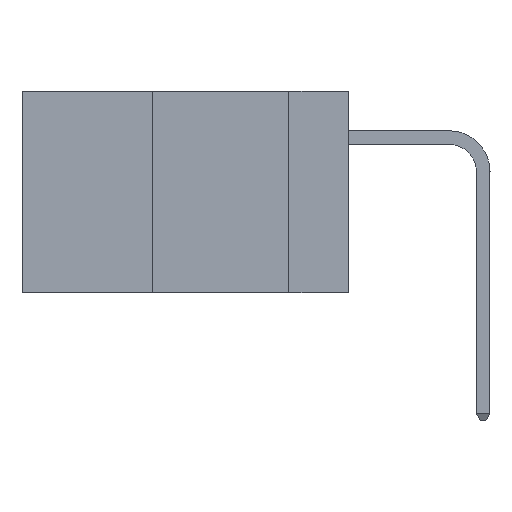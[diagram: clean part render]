
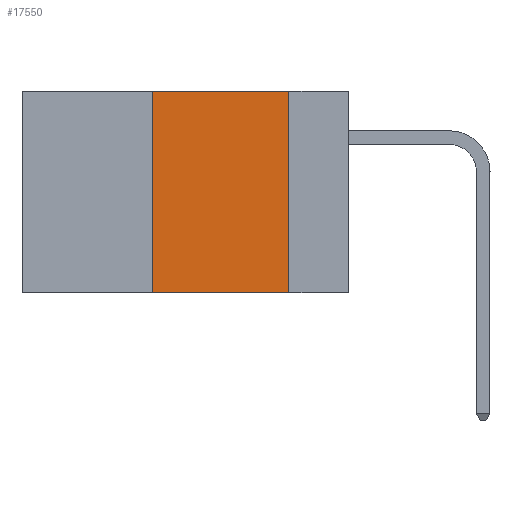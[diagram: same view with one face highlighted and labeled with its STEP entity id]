
A CAD part, left-side view. The second image highlights one B-rep face of the part: STEP entity #17550.
In plain terms, the highlighted planar face has unit normal (-1, 0, 0).
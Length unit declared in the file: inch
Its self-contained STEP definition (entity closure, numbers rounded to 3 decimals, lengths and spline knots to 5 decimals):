
#295 = CARTESIAN_POINT ( 'NONE',  ( 0., 0.6, 0. ) ) ;
#1235 = CARTESIAN_POINT ( 'NONE',  ( 0., 0.11, 0. ) ) ;
#1317 = LINE ( 'NONE', #26488, #11459 ) ;
#2123 = VECTOR ( 'NONE', #9400, 39.37008 ) ;
#2427 = AXIS2_PLACEMENT_3D ( 'NONE', #295, #12502, #10714 ) ;
#2477 = CARTESIAN_POINT ( 'NONE',  ( 0., 0.11, -0.37 ) ) ;
#3123 = CARTESIAN_POINT ( 'NONE',  ( 0., 0.36, 0. ) ) ;
#3642 = CARTESIAN_POINT ( 'NONE',  ( 0., 0.36, -0.37 ) ) ;
#4327 = DIRECTION ( 'NONE',  ( 0., 0., -1. ) ) ;
#4643 = ORIENTED_EDGE ( 'NONE', *, *, #7708, .F. ) ;
#5728 = VERTEX_POINT ( 'NONE', #2477 ) ;
#7194 = ORIENTED_EDGE ( 'NONE', *, *, #15128, .T. ) ;
#7613 = VECTOR ( 'NONE', #17312, 39.37008 ) ;
#7708 = EDGE_CURVE ( 'NONE', #18849, #19179, #10596, .T. ) ;
#8926 = LINE ( 'NONE', #25757, #7613 ) ;
#9400 = DIRECTION ( 'NONE',  ( 0., 0., 1. ) ) ;
#9560 = EDGE_CURVE ( 'NONE', #19179, #5728, #1317, .T. ) ;
#10142 = DIRECTION ( 'NONE',  ( 0., -1., 0. ) ) ;
#10240 = CARTESIAN_POINT ( 'NONE',  ( 0., 0.6, 0. ) ) ;
#10596 = LINE ( 'NONE', #10240, #25767 ) ;
#10714 = DIRECTION ( 'NONE',  ( 0., 0., -1. ) ) ;
#11459 = VECTOR ( 'NONE', #4327, 39.37008 ) ;
#11768 = ORIENTED_EDGE ( 'NONE', *, *, #9560, .F. ) ;
#11888 = VERTEX_POINT ( 'NONE', #3642 ) ;
#12502 = DIRECTION ( 'NONE',  ( 1., 0., 0. ) ) ;
#15128 = EDGE_CURVE ( 'NONE', #11888, #5728, #8926, .T. ) ;
#16936 = FACE_OUTER_BOUND ( 'NONE', #25085, .T. ) ;
#17312 = DIRECTION ( 'NONE',  ( 0., -1., 0. ) ) ;
#17407 = LINE ( 'NONE', #3123, #2123 ) ;
#17550 = ADVANCED_FACE ( 'NONE', ( #16936 ), #24887, .F. ) ;
#18849 = VERTEX_POINT ( 'NONE', #22954 ) ;
#19179 = VERTEX_POINT ( 'NONE', #1235 ) ;
#22390 = EDGE_CURVE ( 'NONE', #11888, #18849, #17407, .T. ) ;
#22954 = CARTESIAN_POINT ( 'NONE',  ( 0., 0.36, 0. ) ) ;
#23325 = ORIENTED_EDGE ( 'NONE', *, *, #22390, .F. ) ;
#24887 = PLANE ( 'NONE',  #2427 ) ;
#25085 = EDGE_LOOP ( 'NONE', ( #11768, #4643, #23325, #7194 ) ) ;
#25757 = CARTESIAN_POINT ( 'NONE',  ( 0., 0.6, -0.37 ) ) ;
#25767 = VECTOR ( 'NONE', #10142, 39.37008 ) ;
#26488 = CARTESIAN_POINT ( 'NONE',  ( 0., 0.11, 0. ) ) ;
